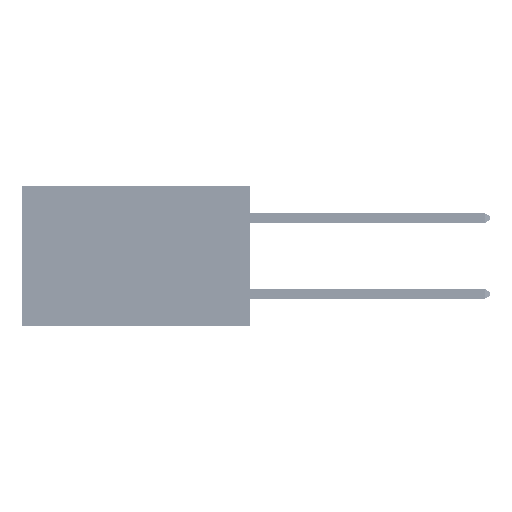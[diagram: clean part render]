
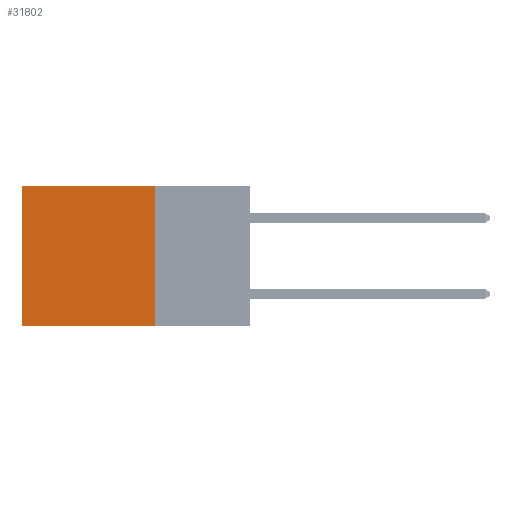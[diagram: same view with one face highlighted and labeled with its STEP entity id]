
A CAD part, left-side view. The second image highlights one B-rep face of the part: STEP entity #31802.
In plain terms, the highlighted planar face has unit normal (-1, 0, 0).
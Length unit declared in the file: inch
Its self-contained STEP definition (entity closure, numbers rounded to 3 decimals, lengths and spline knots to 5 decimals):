
#1673 = CARTESIAN_POINT ( 'NONE',  ( 0.2875, 0.6, 0. ) ) ;
#1824 = ORIENTED_EDGE ( 'NONE', *, *, #12173, .F. ) ;
#2157 = EDGE_CURVE ( 'NONE', #25328, #14768, #14411, .T. ) ;
#4824 = EDGE_CURVE ( 'NONE', #14768, #38789, #10207, .T. ) ;
#5741 = LINE ( 'NONE', #8604, #20921 ) ;
#7268 = CARTESIAN_POINT ( 'NONE',  ( 0.2875, 0.25, 0. ) ) ;
#8604 = CARTESIAN_POINT ( 'NONE',  ( 0.2875, 0.25, 0. ) ) ;
#9070 = CARTESIAN_POINT ( 'NONE',  ( 0.2875, 0.25, 0. ) ) ;
#10207 = LINE ( 'NONE', #13314, #28847 ) ;
#11612 = ORIENTED_EDGE ( 'NONE', *, *, #40989, .F. ) ;
#12173 = EDGE_CURVE ( 'NONE', #25328, #20680, #5741, .T. ) ;
#12617 = EDGE_LOOP ( 'NONE', ( #29214, #11612, #1824, #39130 ) ) ;
#13314 = CARTESIAN_POINT ( 'NONE',  ( 0.2875, 0.6, 0. ) ) ;
#14382 = CARTESIAN_POINT ( 'NONE',  ( 0.2875, 0.25, 0. ) ) ;
#14411 = LINE ( 'NONE', #7268, #44991 ) ;
#14768 = VERTEX_POINT ( 'NONE', #1673 ) ;
#15554 = CARTESIAN_POINT ( 'NONE',  ( 0.2875, 0.25, -0.37 ) ) ;
#15992 = DIRECTION ( 'NONE',  ( 0., 0., -1. ) ) ;
#20680 = VERTEX_POINT ( 'NONE', #26107 ) ;
#20921 = VECTOR ( 'NONE', #15992, 39.37008 ) ;
#21785 = DIRECTION ( 'NONE',  ( 1., 0., 0. ) ) ;
#23653 = LINE ( 'NONE', #15554, #43859 ) ;
#24286 = DIRECTION ( 'NONE',  ( 0., 1., 0. ) ) ;
#25328 = VERTEX_POINT ( 'NONE', #9070 ) ;
#26107 = CARTESIAN_POINT ( 'NONE',  ( 0.2875, 0.25, -0.37 ) ) ;
#27883 = DIRECTION ( 'NONE',  ( 0., 0., -1. ) ) ;
#28847 = VECTOR ( 'NONE', #27883, 39.37008 ) ;
#29214 = ORIENTED_EDGE ( 'NONE', *, *, #4824, .T. ) ;
#31802 = ADVANCED_FACE ( 'NONE', ( #32500 ), #47026, .F. ) ;
#32500 = FACE_OUTER_BOUND ( 'NONE', #12617, .T. ) ;
#34438 = CARTESIAN_POINT ( 'NONE',  ( 0.2875, 0.6, -0.37 ) ) ;
#38789 = VERTEX_POINT ( 'NONE', #34438 ) ;
#39130 = ORIENTED_EDGE ( 'NONE', *, *, #2157, .T. ) ;
#39537 = AXIS2_PLACEMENT_3D ( 'NONE', #14382, #21785, #43451 ) ;
#40175 = DIRECTION ( 'NONE',  ( 0., 1., 0. ) ) ;
#40989 = EDGE_CURVE ( 'NONE', #20680, #38789, #23653, .T. ) ;
#43451 = DIRECTION ( 'NONE',  ( 0., 0., -1. ) ) ;
#43859 = VECTOR ( 'NONE', #40175, 39.37008 ) ;
#44991 = VECTOR ( 'NONE', #24286, 39.37008 ) ;
#47026 = PLANE ( 'NONE',  #39537 ) ;
